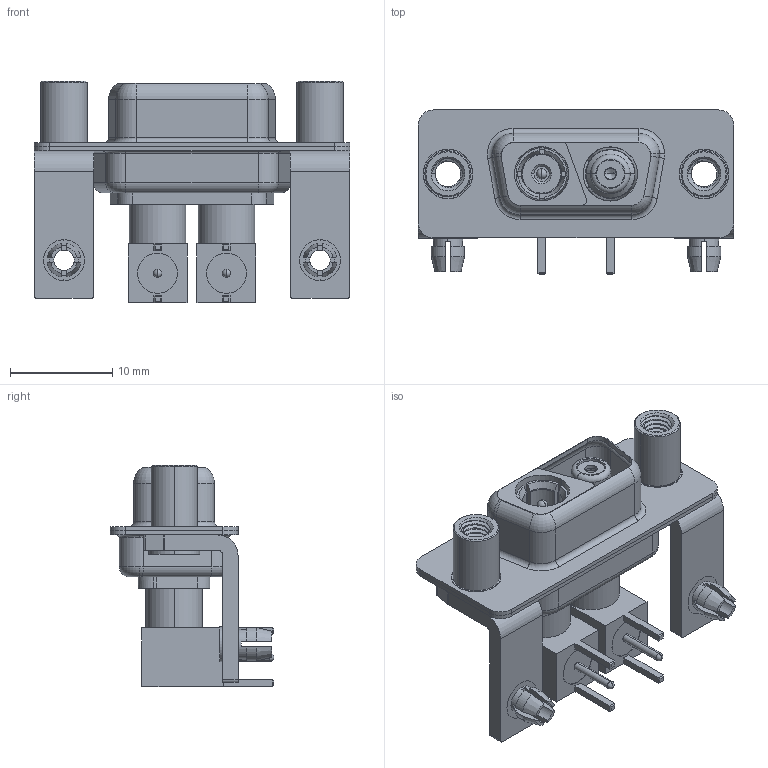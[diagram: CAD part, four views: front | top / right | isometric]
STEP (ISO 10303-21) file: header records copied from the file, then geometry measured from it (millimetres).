
FILE_DESCRIPTION (( 'STEP AP203' ), '1' );
FILE_NAME ('630-2WK2640-7TD.STEP', '2022-05-27T03:55:35', ( '' ), ( '' ), 'SwSTEP 2.0', 'SolidWorks 2020', '' );
FILE_SCHEMA (( 'CONFIG_CONTROL_DESIGN' ));
Length unit declared in the file: millimetre
Products named in the file (19): Pin_RA; Co-Ax Jack_RA PC Tail; 630Combo Shell Rear_09 Contacts; 630Combo Threaded Standoff_D; Insulator Socket; RA Back Shell; Socket_RA; 630Combo Board Lock; Co-Ax Jack Assy_RA; Insulator Socket 2; Co-Ax Plug Assy_RA; Insulator Pin_Straight PC Tail; Locking Collar; Co-Ax Plug_RA PC Tail; 630Combo Housing_2WK2; 630Combo Shell Front_09 Contacts; 630Combo Stabilizer Bracket; Insulator RA Pin; 630-2WK2640-7TD
Assembly tree (24 placements, depth 3):
  630-2WK2640-7TD
    630Combo Housing_2WK2
    630Combo Shell Front_09 Contacts
    630Combo Shell Rear_09 Contacts
    630Combo Stabilizer Bracket  x2
    630Combo Board Lock  x2
    630Combo Threaded Standoff_D  x2
    Co-Ax Plug Assy_RA
      Co-Ax Plug_RA PC Tail
      Insulator Pin_Straight PC Tail
      Pin_RA
      Locking Collar
      RA Back Shell
      Insulator RA Pin
    Co-Ax Jack Assy_RA
      Co-Ax Jack_RA PC Tail
      Insulator Socket
      Insulator Socket 2
      Locking Collar
      Socket_RA
      RA Back Shell
      Insulator RA Pin
Bounding box: 30.8 x 16 x 21.61 mm (x, y, z)
Volume: 2431.3 mm3; surface area: 6702.6 mm2
Topology: 22 solids, 22 shells, 790 faces, 1948 edges, 1231 vertices
Faces by surface type: cylinder 374, plane 261, cone 72, torus 69, bspline 8, sphere 6
Entity records: 22465 total; most frequent: CARTESIAN_POINT 5859, DIRECTION 3219, ORIENTED_EDGE 2914, EDGE_CURVE 1457, AXIS2_PLACEMENT_3D 1294, VERTEX_POINT 925, EDGE_LOOP 684, CIRCLE 664
